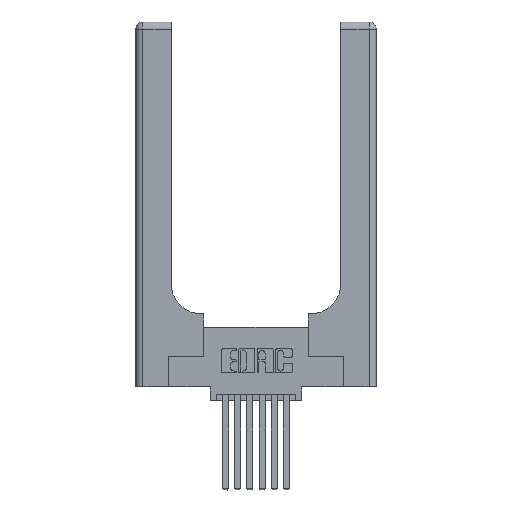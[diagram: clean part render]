
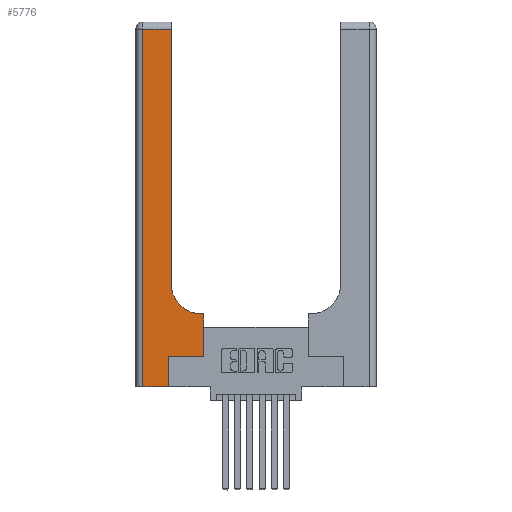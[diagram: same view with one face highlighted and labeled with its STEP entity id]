
A CAD part, top view. The second image highlights one B-rep face of the part: STEP entity #5776.
In plain terms, the highlighted planar face has unit normal (0, 0, 1).
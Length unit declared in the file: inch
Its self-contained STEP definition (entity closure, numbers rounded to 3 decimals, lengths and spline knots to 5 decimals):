
#206 = CARTESIAN_POINT ( 'NONE',  ( 0.5415, 0.85, 0.37 ) ) ;
#519 = VECTOR ( 'NONE', #9796, 39.37008 ) ;
#854 = FACE_OUTER_BOUND ( 'NONE', #8870, .T. ) ;
#964 = EDGE_CURVE ( 'NONE', #14304, #8715, #12523, .T. ) ;
#1223 = CARTESIAN_POINT ( 'NONE',  ( 0.5585, 0.25, 0.37 ) ) ;
#1593 = EDGE_CURVE ( 'NONE', #11322, #14304, #12138, .T. ) ;
#1815 = CARTESIAN_POINT ( 'NONE',  ( 0.5585, 0.25, 0.37 ) ) ;
#1948 = CARTESIAN_POINT ( 'NONE',  ( 0.06, 0., 0.37 ) ) ;
#2223 = DIRECTION ( 'NONE',  ( 0., 1., 0. ) ) ;
#2469 = CARTESIAN_POINT ( 'NONE',  ( 0.5585, 0.6, 0.37 ) ) ;
#2724 = VERTEX_POINT ( 'NONE', #3302 ) ;
#2882 = VECTOR ( 'NONE', #2223, 39.37008 ) ;
#3045 = ORIENTED_EDGE ( 'NONE', *, *, #14033, .T. ) ;
#3302 = CARTESIAN_POINT ( 'NONE',  ( 0.06, 2.94, 0.37 ) ) ;
#3455 = VECTOR ( 'NONE', #6498, 39.37008 ) ;
#3581 = EDGE_CURVE ( 'NONE', #5644, #11322, #8562, .T. ) ;
#3932 = CARTESIAN_POINT ( 'NONE',  ( 0.06, 3., 0.37 ) ) ;
#3950 = VECTOR ( 'NONE', #9194, 39.37008 ) ;
#4119 = VECTOR ( 'NONE', #8847, 39.37008 ) ;
#4367 = ORIENTED_EDGE ( 'NONE', *, *, #12125, .T. ) ;
#4685 = VERTEX_POINT ( 'NONE', #14213 ) ;
#5133 = ORIENTED_EDGE ( 'NONE', *, *, #1593, .T. ) ;
#5361 = CARTESIAN_POINT ( 'NONE',  ( 0.269, 0.25, 0.37 ) ) ;
#5644 = VERTEX_POINT ( 'NONE', #1815 ) ;
#5776 = ADVANCED_FACE ( 'NONE', ( #854 ), #14346, .F. ) ;
#5894 = VECTOR ( 'NONE', #14230, 39.37008 ) ;
#5920 = CARTESIAN_POINT ( 'NONE',  ( 0.2915, 3., 0.37 ) ) ;
#6253 = DIRECTION ( 'NONE',  ( 0., 1., 0. ) ) ;
#6498 = DIRECTION ( 'NONE',  ( -1., 0., 0. ) ) ;
#6524 = LINE ( 'NONE', #3932, #8837 ) ;
#6835 = ORIENTED_EDGE ( 'NONE', *, *, #12366, .T. ) ;
#7618 = CARTESIAN_POINT ( 'NONE',  ( 0., 2.94, 0.37 ) ) ;
#7903 = ORIENTED_EDGE ( 'NONE', *, *, #13082, .T. ) ;
#8148 = DIRECTION ( 'NONE',  ( 1., 0., 0. ) ) ;
#8185 = EDGE_CURVE ( 'NONE', #8201, #2724, #13645, .T. ) ;
#8201 = VERTEX_POINT ( 'NONE', #13193 ) ;
#8363 = VECTOR ( 'NONE', #6253, 39.37008 ) ;
#8562 = LINE ( 'NONE', #1223, #2882 ) ;
#8715 = VERTEX_POINT ( 'NONE', #11239 ) ;
#8837 = VECTOR ( 'NONE', #14128, 39.37008 ) ;
#8845 = DIRECTION ( 'NONE',  ( -1., 0., 0. ) ) ;
#8847 = DIRECTION ( 'NONE',  ( 1., 0., 0. ) ) ;
#8870 = EDGE_LOOP ( 'NONE', ( #6835, #14596, #3045, #10673, #7903, #4367, #11994, #5133, #14188 ) ) ;
#8906 = LINE ( 'NONE', #10751, #5894 ) ;
#9194 = DIRECTION ( 'NONE',  ( 0., 1., 0. ) ) ;
#9796 = DIRECTION ( 'NONE',  ( -1., 0., 0. ) ) ;
#10125 = LINE ( 'NONE', #12016, #4119 ) ;
#10238 = CARTESIAN_POINT ( 'NONE',  ( 0.5415, 0.6, 0.37 ) ) ;
#10673 = ORIENTED_EDGE ( 'NONE', *, *, #12555, .T. ) ;
#10751 = CARTESIAN_POINT ( 'NONE',  ( 0., 0., 0.37 ) ) ;
#11175 = LINE ( 'NONE', #5920, #3950 ) ;
#11239 = CARTESIAN_POINT ( 'NONE',  ( 0.2915, 0.85, 0.37 ) ) ;
#11322 = VERTEX_POINT ( 'NONE', #2469 ) ;
#11606 = DIRECTION ( 'NONE',  ( 0., 0., -1. ) ) ;
#11994 = ORIENTED_EDGE ( 'NONE', *, *, #3581, .T. ) ;
#12016 = CARTESIAN_POINT ( 'NONE',  ( 0.269, 0.25, 0.37 ) ) ;
#12125 = EDGE_CURVE ( 'NONE', #13861, #5644, #10125, .T. ) ;
#12138 = LINE ( 'NONE', #12277, #3455 ) ;
#12158 = CARTESIAN_POINT ( 'NONE',  ( 0., 3., 0.37 ) ) ;
#12203 = DIRECTION ( 'NONE',  ( 0., 0., -1. ) ) ;
#12277 = CARTESIAN_POINT ( 'NONE',  ( 0.2915, 0.6, 0.37 ) ) ;
#12366 = EDGE_CURVE ( 'NONE', #8715, #8201, #11175, .T. ) ;
#12428 = LINE ( 'NONE', #12955, #8363 ) ;
#12523 = CIRCLE ( 'NONE', #13950, 0.25 ) ;
#12526 = AXIS2_PLACEMENT_3D ( 'NONE', #12158, #12203, #8845 ) ;
#12555 = EDGE_CURVE ( 'NONE', #14575, #4685, #8906, .T. ) ;
#12955 = CARTESIAN_POINT ( 'NONE',  ( 0.269, 0., 0.37 ) ) ;
#13082 = EDGE_CURVE ( 'NONE', #4685, #13861, #12428, .T. ) ;
#13193 = CARTESIAN_POINT ( 'NONE',  ( 0.2915, 2.94, 0.37 ) ) ;
#13645 = LINE ( 'NONE', #7618, #519 ) ;
#13861 = VERTEX_POINT ( 'NONE', #5361 ) ;
#13950 = AXIS2_PLACEMENT_3D ( 'NONE', #206, #11606, #8148 ) ;
#14033 = EDGE_CURVE ( 'NONE', #2724, #14575, #6524, .T. ) ;
#14128 = DIRECTION ( 'NONE',  ( 0., -1., 0. ) ) ;
#14188 = ORIENTED_EDGE ( 'NONE', *, *, #964, .T. ) ;
#14213 = CARTESIAN_POINT ( 'NONE',  ( 0.269, 0., 0.37 ) ) ;
#14230 = DIRECTION ( 'NONE',  ( 1., 0., 0. ) ) ;
#14304 = VERTEX_POINT ( 'NONE', #10238 ) ;
#14346 = PLANE ( 'NONE',  #12526 ) ;
#14575 = VERTEX_POINT ( 'NONE', #1948 ) ;
#14596 = ORIENTED_EDGE ( 'NONE', *, *, #8185, .T. ) ;
